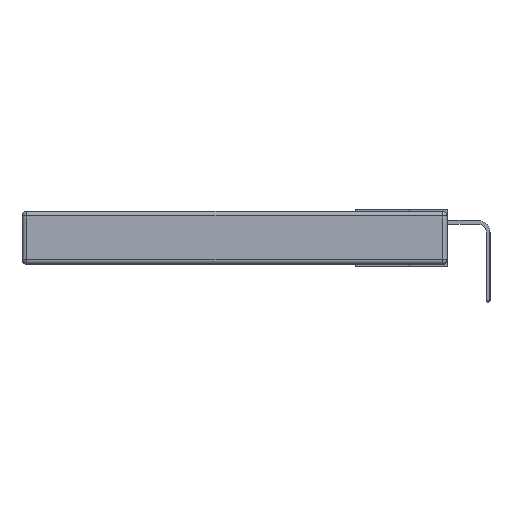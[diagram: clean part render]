
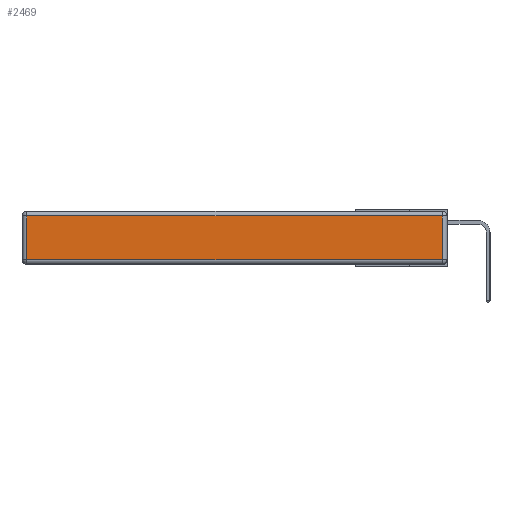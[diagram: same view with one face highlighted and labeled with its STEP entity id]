
A CAD part, left-side view. The second image highlights one B-rep face of the part: STEP entity #2469.
In plain terms, the highlighted planar face has unit normal (-1, 0, 0).
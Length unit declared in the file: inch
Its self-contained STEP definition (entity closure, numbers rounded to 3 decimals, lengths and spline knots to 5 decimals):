
#16 = CARTESIAN_POINT ( 'NONE',  ( 0., 0., -0.313 ) ) ;
#407 = VERTEX_POINT ( 'NONE', #5305 ) ;
#1551 = VERTEX_POINT ( 'NONE', #7045 ) ;
#1579 = EDGE_CURVE ( 'NONE', #7524, #2105, #6170, .T. ) ;
#2105 = VERTEX_POINT ( 'NONE', #16422 ) ;
#2469 = ADVANCED_FACE ( 'NONE', ( #21335 ), #20806, .T. ) ;
#2849 = DIRECTION ( 'NONE',  ( 0., -1., 0. ) ) ;
#2980 = VECTOR ( 'NONE', #19187, 39.37008 ) ;
#4146 = DIRECTION ( 'NONE',  ( 0., 0., -1. ) ) ;
#5305 = CARTESIAN_POINT ( 'NONE',  ( 0., 0.03, -0.03 ) ) ;
#6170 = LINE ( 'NONE', #32592, #27148 ) ;
#7045 = CARTESIAN_POINT ( 'NONE',  ( 0., 0.03, -0.313 ) ) ;
#7524 = VERTEX_POINT ( 'NONE', #9496 ) ;
#7738 = EDGE_CURVE ( 'NONE', #2105, #1551, #12502, .T. ) ;
#7996 = ORIENTED_EDGE ( 'NONE', *, *, #25552, .T. ) ;
#9496 = CARTESIAN_POINT ( 'NONE',  ( 0., 2.72, -0.03 ) ) ;
#10298 = CARTESIAN_POINT ( 'NONE',  ( 0., 0., -0.343 ) ) ;
#10511 = LINE ( 'NONE', #32803, #14579 ) ;
#12502 = LINE ( 'NONE', #16, #17787 ) ;
#14344 = CARTESIAN_POINT ( 'NONE',  ( 0., 0.03, -0.343 ) ) ;
#14579 = VECTOR ( 'NONE', #30553, 39.37008 ) ;
#16422 = CARTESIAN_POINT ( 'NONE',  ( 0., 2.72, -0.313 ) ) ;
#17317 = ORIENTED_EDGE ( 'NONE', *, *, #1579, .T. ) ;
#17787 = VECTOR ( 'NONE', #2849, 39.37008 ) ;
#18456 = DIRECTION ( 'NONE',  ( -1., 0., 0. ) ) ;
#18958 = EDGE_CURVE ( 'NONE', #407, #7524, #10511, .T. ) ;
#19187 = DIRECTION ( 'NONE',  ( 0., 0., 1. ) ) ;
#20806 = PLANE ( 'NONE',  #30788 ) ;
#21335 = FACE_OUTER_BOUND ( 'NONE', #25303, .T. ) ;
#21508 = ORIENTED_EDGE ( 'NONE', *, *, #7738, .T. ) ;
#21925 = LINE ( 'NONE', #14344, #2980 ) ;
#25303 = EDGE_LOOP ( 'NONE', ( #21508, #7996, #26004, #17317 ) ) ;
#25552 = EDGE_CURVE ( 'NONE', #1551, #407, #21925, .T. ) ;
#26004 = ORIENTED_EDGE ( 'NONE', *, *, #18958, .T. ) ;
#27148 = VECTOR ( 'NONE', #4146, 39.37008 ) ;
#28360 = DIRECTION ( 'NONE',  ( 0., 0., 1. ) ) ;
#30553 = DIRECTION ( 'NONE',  ( 0., 1., 0. ) ) ;
#30788 = AXIS2_PLACEMENT_3D ( 'NONE', #10298, #18456, #28360 ) ;
#32592 = CARTESIAN_POINT ( 'NONE',  ( 0., 2.72, -0.343 ) ) ;
#32803 = CARTESIAN_POINT ( 'NONE',  ( 0., 2.75, -0.03 ) ) ;
